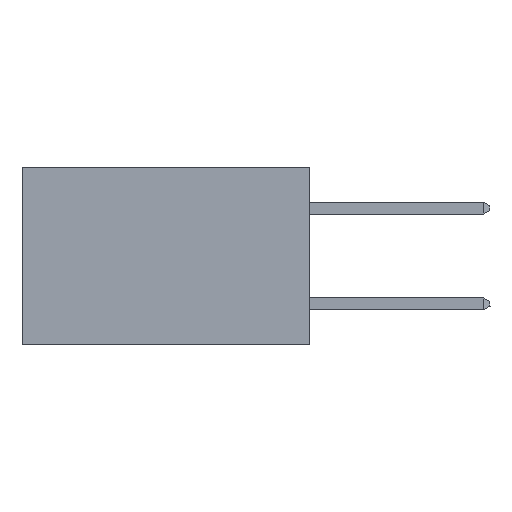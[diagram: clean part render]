
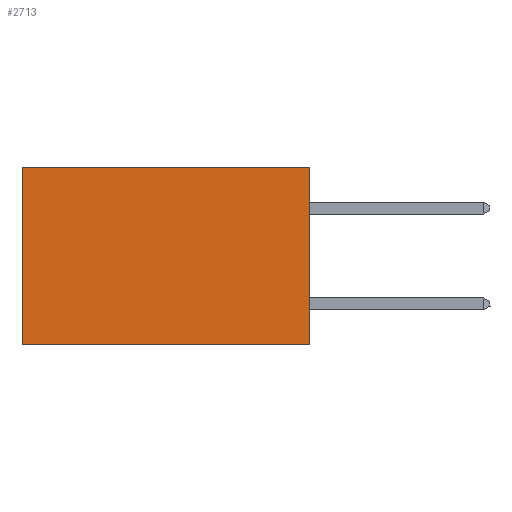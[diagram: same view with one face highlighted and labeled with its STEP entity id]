
A CAD part, left-side view. The second image highlights one B-rep face of the part: STEP entity #2713.
In plain terms, the highlighted planar face has unit normal (-1, 0, 0).
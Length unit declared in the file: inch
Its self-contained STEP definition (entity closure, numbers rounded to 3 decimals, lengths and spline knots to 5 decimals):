
#455 = VECTOR ( 'NONE', #10451, 39.37008 ) ;
#1437 = VERTEX_POINT ( 'NONE', #23063 ) ;
#1979 = EDGE_CURVE ( 'NONE', #17903, #1437, #10198, .T. ) ;
#2298 = DIRECTION ( 'NONE',  ( 0., 0., -1. ) ) ;
#2713 = ADVANCED_FACE ( 'NONE', ( #6617 ), #7862, .F. ) ;
#3513 = LINE ( 'NONE', #9717, #16641 ) ;
#3866 = LINE ( 'NONE', #8512, #5031 ) ;
#4175 = EDGE_CURVE ( 'NONE', #4679, #5350, #4235, .T. ) ;
#4235 = LINE ( 'NONE', #19673, #455 ) ;
#4629 = CARTESIAN_POINT ( 'NONE',  ( 0.2875, 0., 0. ) ) ;
#4679 = VERTEX_POINT ( 'NONE', #4629 ) ;
#5031 = VECTOR ( 'NONE', #12760, 39.37008 ) ;
#5201 = VECTOR ( 'NONE', #19740, 39.37008 ) ;
#5350 = VERTEX_POINT ( 'NONE', #9935 ) ;
#5960 = ORIENTED_EDGE ( 'NONE', *, *, #12352, .T. ) ;
#6617 = FACE_OUTER_BOUND ( 'NONE', #24243, .T. ) ;
#7862 = PLANE ( 'NONE',  #15517 ) ;
#8512 = CARTESIAN_POINT ( 'NONE',  ( 0.2875, 0., -0.37 ) ) ;
#9717 = CARTESIAN_POINT ( 'NONE',  ( 0.2875, 0., 0. ) ) ;
#9935 = CARTESIAN_POINT ( 'NONE',  ( 0.2875, 0., -0.37 ) ) ;
#10198 = LINE ( 'NONE', #21710, #5201 ) ;
#10451 = DIRECTION ( 'NONE',  ( 0., 0., -1. ) ) ;
#11763 = DIRECTION ( 'NONE',  ( 1., 0., 0. ) ) ;
#12014 = ORIENTED_EDGE ( 'NONE', *, *, #4175, .F. ) ;
#12352 = EDGE_CURVE ( 'NONE', #4679, #17903, #3513, .T. ) ;
#12760 = DIRECTION ( 'NONE',  ( 0., 1., 0. ) ) ;
#15517 = AXIS2_PLACEMENT_3D ( 'NONE', #22857, #11763, #2298 ) ;
#16641 = VECTOR ( 'NONE', #22810, 39.37008 ) ;
#17529 = ORIENTED_EDGE ( 'NONE', *, *, #21330, .F. ) ;
#17903 = VERTEX_POINT ( 'NONE', #18122 ) ;
#17967 = ORIENTED_EDGE ( 'NONE', *, *, #1979, .T. ) ;
#18122 = CARTESIAN_POINT ( 'NONE',  ( 0.2875, 0.6, 0. ) ) ;
#19673 = CARTESIAN_POINT ( 'NONE',  ( 0.2875, 0., 0. ) ) ;
#19740 = DIRECTION ( 'NONE',  ( 0., 0., -1. ) ) ;
#21330 = EDGE_CURVE ( 'NONE', #5350, #1437, #3866, .T. ) ;
#21710 = CARTESIAN_POINT ( 'NONE',  ( 0.2875, 0.6, 0. ) ) ;
#22810 = DIRECTION ( 'NONE',  ( 0., 1., 0. ) ) ;
#22857 = CARTESIAN_POINT ( 'NONE',  ( 0.2875, 0., 0. ) ) ;
#23063 = CARTESIAN_POINT ( 'NONE',  ( 0.2875, 0.6, -0.37 ) ) ;
#24243 = EDGE_LOOP ( 'NONE', ( #17967, #17529, #12014, #5960 ) ) ;
